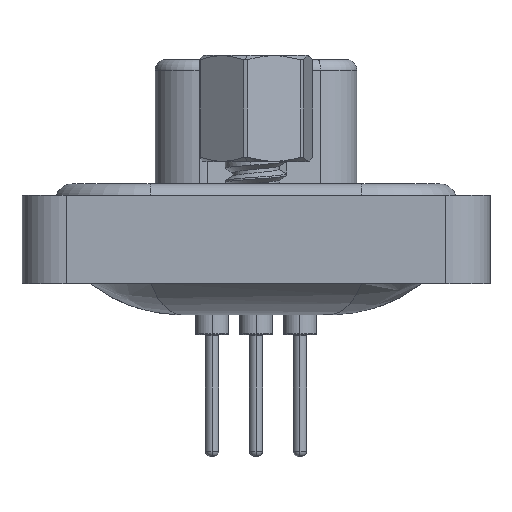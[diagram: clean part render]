
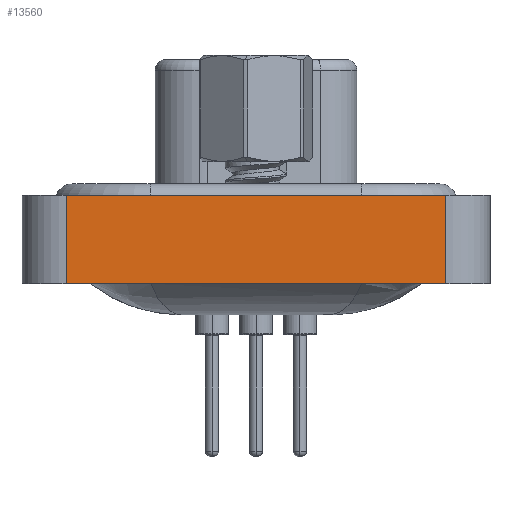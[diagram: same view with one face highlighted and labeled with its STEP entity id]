
A CAD part, left-side view. The second image highlights one B-rep face of the part: STEP entity #13560.
In plain terms, the highlighted planar face has unit normal (-1, 0, 0).
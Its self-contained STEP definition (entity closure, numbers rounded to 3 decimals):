
#165 = CARTESIAN_POINT ( 'NONE',  ( -7.26, -8.55, -3.6 ) ) ;
#318 = CARTESIAN_POINT ( 'NONE',  ( -7.26, 8.55, 0.4 ) ) ;
#800 = EDGE_CURVE ( 'NONE', #10195, #20084, #19367, .T. ) ;
#807 = EDGE_CURVE ( 'NONE', #10195, #10411, #17637, .T. ) ;
#1144 = VERTEX_POINT ( 'NONE', #14000 ) ;
#2192 = DIRECTION ( 'NONE',  ( 0., -1., 0. ) ) ;
#2656 = ORIENTED_EDGE ( 'NONE', *, *, #807, .F. ) ;
#2992 = ORIENTED_EDGE ( 'NONE', *, *, #9879, .F. ) ;
#3369 = AXIS2_PLACEMENT_3D ( 'NONE', #165, #10481, #5383 ) ;
#5383 = DIRECTION ( 'NONE',  ( 0., 0., 1. ) ) ;
#5515 = DIRECTION ( 'NONE',  ( 0., 0., 1. ) ) ;
#5868 = VECTOR ( 'NONE', #2192, 1000. ) ;
#6358 = VECTOR ( 'NONE', #20208, 1000. ) ;
#6448 = EDGE_LOOP ( 'NONE', ( #9220, #2992, #2656, #16878 ) ) ;
#7862 = CARTESIAN_POINT ( 'NONE',  ( -7.26, -8.55, -3.6 ) ) ;
#8806 = CARTESIAN_POINT ( 'NONE',  ( -7.26, -8.55, 0.4 ) ) ;
#9017 = VECTOR ( 'NONE', #5515, 1000. ) ;
#9220 = ORIENTED_EDGE ( 'NONE', *, *, #16128, .T. ) ;
#9879 = EDGE_CURVE ( 'NONE', #10411, #1144, #10653, .T. ) ;
#10195 = VERTEX_POINT ( 'NONE', #13843 ) ;
#10411 = VERTEX_POINT ( 'NONE', #318 ) ;
#10481 = DIRECTION ( 'NONE',  ( -1., 0., 0. ) ) ;
#10653 = LINE ( 'NONE', #8806, #5868 ) ;
#13560 = ADVANCED_FACE ( 'NONE', ( #15545 ), #19128, .T. ) ;
#13843 = CARTESIAN_POINT ( 'NONE',  ( -7.26, 8.55, -3.6 ) ) ;
#14000 = CARTESIAN_POINT ( 'NONE',  ( -7.26, -8.55, 0.4 ) ) ;
#15545 = FACE_OUTER_BOUND ( 'NONE', #6448, .T. ) ;
#16127 = DIRECTION ( 'NONE',  ( 0., -1., 0. ) ) ;
#16128 = EDGE_CURVE ( 'NONE', #20084, #1144, #17203, .T. ) ;
#16172 = CARTESIAN_POINT ( 'NONE',  ( -7.26, -8.55, -3.6 ) ) ;
#16878 = ORIENTED_EDGE ( 'NONE', *, *, #800, .T. ) ;
#17203 = LINE ( 'NONE', #7862, #6358 ) ;
#17637 = LINE ( 'NONE', #17750, #9017 ) ;
#17750 = CARTESIAN_POINT ( 'NONE',  ( -7.26, 8.55, -3.6 ) ) ;
#17868 = CARTESIAN_POINT ( 'NONE',  ( -7.26, -8.55, -3.6 ) ) ;
#18962 = VECTOR ( 'NONE', #16127, 1000. ) ;
#19128 = PLANE ( 'NONE',  #3369 ) ;
#19367 = LINE ( 'NONE', #17868, #18962 ) ;
#20084 = VERTEX_POINT ( 'NONE', #16172 ) ;
#20208 = DIRECTION ( 'NONE',  ( 0., 0., 1. ) ) ;
